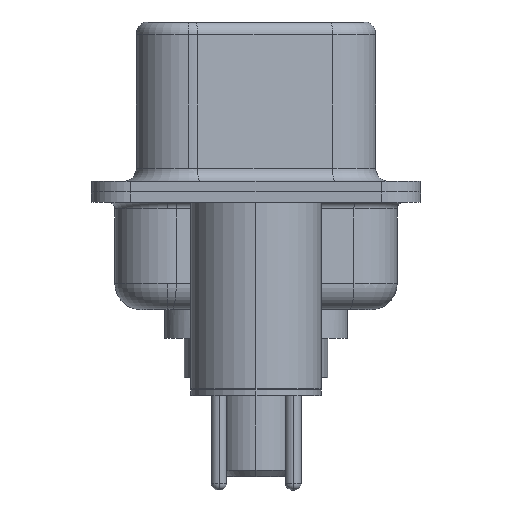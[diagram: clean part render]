
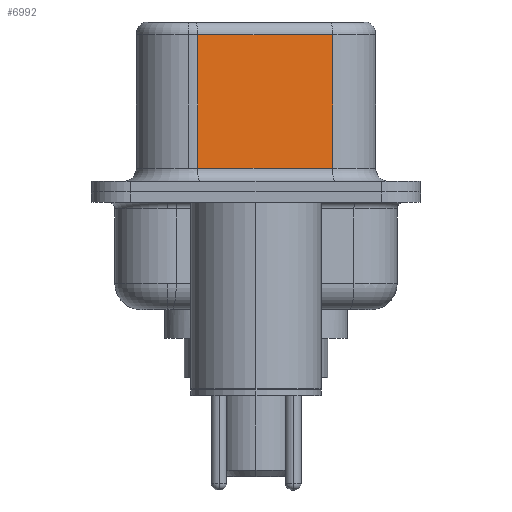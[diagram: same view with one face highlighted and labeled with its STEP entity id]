
A CAD part, left-side view. The second image highlights one B-rep face of the part: STEP entity #6992.
In plain terms, the highlighted planar face has unit normal (-0.985, -0.174, 0).
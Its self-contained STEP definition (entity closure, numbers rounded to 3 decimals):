
#736 = ORIENTED_EDGE ( 'NONE', *, *, #8135, .T. ) ;
#1175 = DIRECTION ( 'NONE',  ( -0.174, 0.985, 0. ) ) ;
#1376 = ORIENTED_EDGE ( 'NONE', *, *, #16020, .T. ) ;
#2040 = VECTOR ( 'NONE', #1175, 1000. ) ;
#2583 = LINE ( 'NONE', #20402, #2040 ) ;
#3225 = CARTESIAN_POINT ( 'NONE',  ( 4.565, -2.927, 0.9 ) ) ;
#3757 = DIRECTION ( 'NONE',  ( -0.174, 0.985, 0. ) ) ;
#3809 = DIRECTION ( 'NONE',  ( 0.985, 0.174, 0. ) ) ;
#3825 = CARTESIAN_POINT ( 'NONE',  ( 4.565, -2.927, 0.9 ) ) ;
#4119 = PLANE ( 'NONE',  #6708 ) ;
#4298 = CARTESIAN_POINT ( 'NONE',  ( 4.565, -2.927, 6.52 ) ) ;
#5175 = DIRECTION ( 'NONE',  ( 0.174, -0.985, 0. ) ) ;
#5655 = ORIENTED_EDGE ( 'NONE', *, *, #6765, .F. ) ;
#5725 = EDGE_CURVE ( 'NONE', #17200, #21107, #20321, .T. ) ;
#6407 = CARTESIAN_POINT ( 'NONE',  ( 3.655, 2.233, 6.52 ) ) ;
#6554 = CARTESIAN_POINT ( 'NONE',  ( 4.565, -2.927, 6.02 ) ) ;
#6689 = VERTEX_POINT ( 'NONE', #7207 ) ;
#6708 = AXIS2_PLACEMENT_3D ( 'NONE', #4298, #3809, #3757 ) ;
#6765 = EDGE_CURVE ( 'NONE', #11686, #21107, #17102, .T. ) ;
#6992 = ADVANCED_FACE ( 'NONE', ( #17352 ), #4119, .F. ) ;
#7207 = CARTESIAN_POINT ( 'NONE',  ( 3.655, 2.233, 6.02 ) ) ;
#7618 = VECTOR ( 'NONE', #13405, 1000. ) ;
#8135 = EDGE_CURVE ( 'NONE', #11686, #6689, #2583, .T. ) ;
#8504 = ORIENTED_EDGE ( 'NONE', *, *, #5725, .T. ) ;
#8699 = VECTOR ( 'NONE', #14853, 1000. ) ;
#8819 = CARTESIAN_POINT ( 'NONE',  ( 3.655, 2.233, 0.9 ) ) ;
#9203 = LINE ( 'NONE', #6407, #8699 ) ;
#11686 = VERTEX_POINT ( 'NONE', #6554 ) ;
#13158 = CARTESIAN_POINT ( 'NONE',  ( 4.565, -2.927, 6.52 ) ) ;
#13405 = DIRECTION ( 'NONE',  ( 0., 0., -1. ) ) ;
#14853 = DIRECTION ( 'NONE',  ( 0., 0., -1. ) ) ;
#15562 = VECTOR ( 'NONE', #5175, 1000. ) ;
#16020 = EDGE_CURVE ( 'NONE', #6689, #17200, #9203, .T. ) ;
#17102 = LINE ( 'NONE', #13158, #7618 ) ;
#17200 = VERTEX_POINT ( 'NONE', #8819 ) ;
#17352 = FACE_OUTER_BOUND ( 'NONE', #19509, .T. ) ;
#19509 = EDGE_LOOP ( 'NONE', ( #5655, #736, #1376, #8504 ) ) ;
#20321 = LINE ( 'NONE', #3825, #15562 ) ;
#20402 = CARTESIAN_POINT ( 'NONE',  ( 4.565, -2.927, 6.02 ) ) ;
#21107 = VERTEX_POINT ( 'NONE', #3225 ) ;
